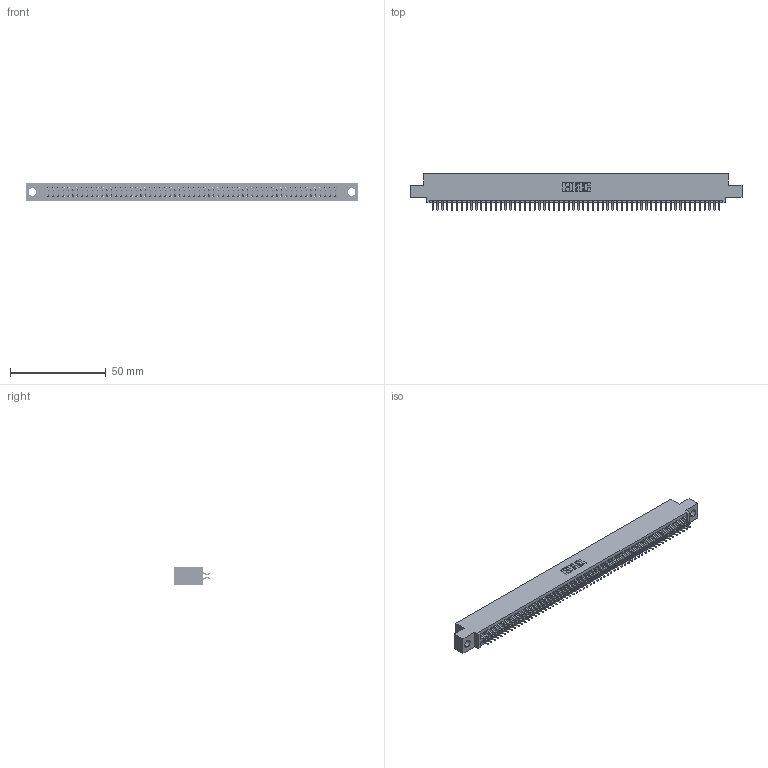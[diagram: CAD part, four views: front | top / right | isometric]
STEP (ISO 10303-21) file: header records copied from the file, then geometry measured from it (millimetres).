
FILE_DESCRIPTION (( 'STEP AP203' ), '1' );
FILE_NAME ('845-120-556-504.STEP', '2018-11-21T05:53:33', ( '' ), ( '' ), 'SwSTEP 2.0', 'SolidWorks 2016', '' );
FILE_SCHEMA (( 'CONFIG_CONTROL_DESIGN' ));
Length unit declared in the file: inch
Products named in the file (3): 845-120-556-504; 845 Part_0.110 Offset - 0.156 Dia-TH; 345-292-001_556 Tail
Assembly tree (121 placements, depth 2):
  845-120-556-504
    845 Part_0.110 Offset - 0.156 Dia-TH
    345-292-001_556 Tail  x120
Bounding box: 173.61 x 19.24 x 9.4 mm (x, y, z)
Volume: 16865.7 mm3; surface area: 25081.9 mm2
Topology: 121 solids, 121 shells, 6850 faces, 20393 edges, 13434 vertices
Faces by surface type: plane 4524, cylinder 2326
Entity records: 45009 total; most frequent: CARTESIAN_POINT 7544, ORIENTED_EDGE 7466, DIRECTION 6617, EDGE_CURVE 3733, VECTOR 3353, LINE 3353, VERTEX_POINT 2486, AXIS2_PLACEMENT_3D 1632
